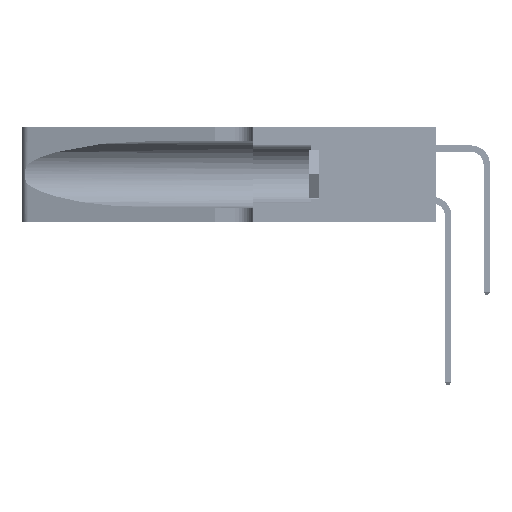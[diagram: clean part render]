
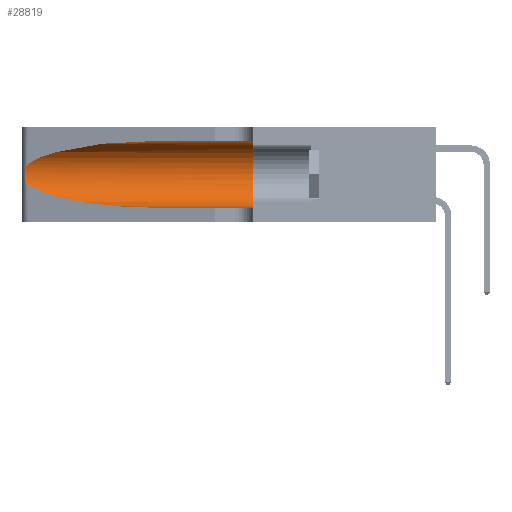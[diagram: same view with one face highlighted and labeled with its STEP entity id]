
A CAD part, left-side view. The second image highlights one B-rep face of the part: STEP entity #28819.
In plain terms, the highlighted cylindrical face has radius 3.308 mm (diameter 6.617 mm), a partial arc.
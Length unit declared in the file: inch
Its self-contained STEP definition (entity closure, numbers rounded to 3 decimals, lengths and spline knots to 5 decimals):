
#1353 = CARTESIAN_POINT ( 'NONE',  ( 0.1305, 0.72297, 0.05475 ) ) ;
#1608 = CARTESIAN_POINT ( 'NONE',  ( 0.25639, 1.23186, 0.15144 ) ) ;
#2017 = CARTESIAN_POINT ( 'NONE',  ( 0.1305, 0.35, 0.31525 ) ) ;
#2249 = ORIENTED_EDGE ( 'NONE', *, *, #4533, .F. ) ;
#2928 = DIRECTION ( 'NONE',  ( 0., 0., -1. ) ) ;
#4365 = CARTESIAN_POINT ( 'NONE',  ( 0.2373, 1.15595, 0.08982 ) ) ;
#4533 = EDGE_CURVE ( 'NONE', #17138, #28572, #42038, .T. ) ;
#5854 = CARTESIAN_POINT ( 'NONE',  ( 0.25487, 1.22718, 0.14631 ) ) ;
#6429 = EDGE_CURVE ( 'NONE', #27896, #28572, #28054, .T. ) ;
#7450 = ORIENTED_EDGE ( 'NONE', *, *, #48011, .T. ) ;
#9872 = CARTESIAN_POINT ( 'NONE',  ( 0.25639, 1.23184, 0.21858 ) ) ;
#12907 = CARTESIAN_POINT ( 'NONE',  ( 0.1305, 1.61858, 0.31525 ) ) ;
#14051 = CARTESIAN_POINT ( 'NONE',  ( 0.25854, 1.2359, 0.20912 ) ) ;
#16298 = AXIS2_PLACEMENT_3D ( 'NONE', #24358, #53357, #28524 ) ;
#16962 = CARTESIAN_POINT ( 'NONE',  ( 0.1305, 0.72297, 0.05475 ) ) ;
#17138 = VERTEX_POINT ( 'NONE', #2017 ) ;
#18266 = CARTESIAN_POINT ( 'NONE',  ( 0.26075, 1.23896, 0.19203 ) ) ;
#20744 = CARTESIAN_POINT ( 'NONE',  ( 0.25487, 1.22718, 0.22369 ) ) ;
#20755 = CYLINDRICAL_SURFACE ( 'NONE', #26564, 0.13025 ) ;
#20875 = ORIENTED_EDGE ( 'NONE', *, *, #33812, .T. ) ;
#22387 = CARTESIAN_POINT ( 'NONE',  ( 0.26017, 1.23833, 0.17102 ) ) ;
#23484 = EDGE_LOOP ( 'NONE', ( #20875, #49934, #7450, #38421, #2249, #41766 ) ) ;
#24358 = CARTESIAN_POINT ( 'NONE',  ( 0.1305, 0.35, 0.185 ) ) ;
#26370 = CARTESIAN_POINT ( 'NONE',  ( 0.25555, 1.22994, 0.2215 ) ) ;
#26554 = CARTESIAN_POINT ( 'NONE',  ( 0.25789, 1.23486, 0.15765 ) ) ;
#26564 = AXIS2_PLACEMENT_3D ( 'NONE', #48472, #31990, #2928 ) ;
#27896 = VERTEX_POINT ( 'NONE', #1353 ) ;
#28054 = LINE ( 'NONE', #49598, #48800 ) ;
#28524 = DIRECTION ( 'NONE',  ( 0., 0., 1. ) ) ;
#28572 = VERTEX_POINT ( 'NONE', #46867 ) ;
#28819 = ADVANCED_FACE ( 'NONE', ( #42798 ), #20755, .F. ) ;
#28870 = CARTESIAN_POINT ( 'NONE',  ( 0.1305, 0.72297, 0.31525 ) ) ;
#28943 = VERTEX_POINT ( 'NONE', #32700 ) ;
#29731 = EDGE_CURVE ( 'NONE', #28943, #17138, #52408, .T. ) ;
#30706 = CARTESIAN_POINT ( 'NONE',  ( 0.25555, 1.22993, 0.14849 ) ) ;
#31990 = DIRECTION ( 'NONE',  ( 0., -1., 0. ) ) ;
#32700 = CARTESIAN_POINT ( 'NONE',  ( 0.1305, 0.72297, 0.31525 ) ) ;
#33095 = DIRECTION ( 'NONE',  ( 0., -1., 0. ) ) ;
#33812 = EDGE_CURVE ( 'NONE', #28943, #36683, #44783, .T. ) ;
#36683 = VERTEX_POINT ( 'NONE', #49891 ) ;
#37570 = CARTESIAN_POINT ( 'NONE',  ( 0.25487, 1.22718, 0.14631 ) ) ;
#38421 = ORIENTED_EDGE ( 'NONE', *, *, #6429, .T. ) ;
#38883 = CARTESIAN_POINT ( 'NONE',  ( 0.25787, 1.23484, 0.2124 ) ) ;
#39419 = VERTEX_POINT ( 'NONE', #40006 ) ;
#40006 = CARTESIAN_POINT ( 'NONE',  ( 0.25487, 1.22718, 0.14631 ) ) ;
#40807 = B_SPLINE_CURVE_WITH_KNOTS ( 'NONE', 3,
 ( #51202, #26370, #9872, #38883, #14051, #43045, #18266, #47182, #22387, #51382, #26554, #1608, #30706, #5854 ),
 .UNSPECIFIED., .F., .F.,
 ( 4, 2, 2, 2, 2, 2, 4 ),
 ( 0., 0.00027, 0.00053, 0.00107, 0.0016, 0.00187, 0.00214 ),
 .UNSPECIFIED. ) ;
#41384 = VECTOR ( 'NONE', #41902, 39.37008 ) ;
#41759 = CARTESIAN_POINT ( 'NONE',  ( 0.18966, 0.96281, 0.05475 ) ) ;
#41766 = ORIENTED_EDGE ( 'NONE', *, *, #29731, .F. ) ;
#41902 = DIRECTION ( 'NONE',  ( 0., -1., 0. ) ) ;
#42038 = CIRCLE ( 'NONE', #16298, 0.13025 ) ;
#42798 = FACE_OUTER_BOUND ( 'NONE', #23484, .T. ) ;
#43045 = CARTESIAN_POINT ( 'NONE',  ( 0.26018, 1.23835, 0.19895 ) ) ;
#44783 =( BOUNDED_CURVE ( )  B_SPLINE_CURVE ( 3, ( #28870, #53714, #45528, #20744 ),
 .UNSPECIFIED., .F., .T. ) 
 B_SPLINE_CURVE_WITH_KNOTS ( ( 4, 4 ),
 ( 1.5708, 2.84003 ),
 .UNSPECIFIED. ) 
 CURVE ( )  GEOMETRIC_REPRESENTATION_ITEM ( )  RATIONAL_B_SPLINE_CURVE ( ( 1., 0.87, 0.87, 1. ) ) 
 REPRESENTATION_ITEM ( '' )  );
#45528 = CARTESIAN_POINT ( 'NONE',  ( 0.2373, 1.15595, 0.28018 ) ) ;
#46867 = CARTESIAN_POINT ( 'NONE',  ( 0.1305, 0.35, 0.05475 ) ) ;
#47182 = CARTESIAN_POINT ( 'NONE',  ( 0.26075, 1.23896, 0.178 ) ) ;
#48011 = EDGE_CURVE ( 'NONE', #39419, #27896, #50439, .T. ) ;
#48472 = CARTESIAN_POINT ( 'NONE',  ( 0.1305, 1.61858, 0.185 ) ) ;
#48800 = VECTOR ( 'NONE', #33095, 39.37008 ) ;
#49598 = CARTESIAN_POINT ( 'NONE',  ( 0.1305, 1.61858, 0.05475 ) ) ;
#49891 = CARTESIAN_POINT ( 'NONE',  ( 0.25487, 1.22718, 0.22369 ) ) ;
#49897 = EDGE_CURVE ( 'NONE', #36683, #39419, #40807, .T. ) ;
#49934 = ORIENTED_EDGE ( 'NONE', *, *, #49897, .T. ) ;
#50439 =( BOUNDED_CURVE ( )  B_SPLINE_CURVE ( 3, ( #37570, #4365, #41759, #16962 ),
 .UNSPECIFIED., .F., .F. ) 
 B_SPLINE_CURVE_WITH_KNOTS ( ( 4, 4 ),
 ( 3.44316, 4.71239 ),
 .UNSPECIFIED. ) 
 CURVE ( )  GEOMETRIC_REPRESENTATION_ITEM ( )  RATIONAL_B_SPLINE_CURVE ( ( 1., 0.87, 0.87, 1. ) ) 
 REPRESENTATION_ITEM ( '' )  );
#51202 = CARTESIAN_POINT ( 'NONE',  ( 0.25487, 1.22718, 0.22369 ) ) ;
#51382 = CARTESIAN_POINT ( 'NONE',  ( 0.25856, 1.23593, 0.16098 ) ) ;
#52408 = LINE ( 'NONE', #12907, #41384 ) ;
#53357 = DIRECTION ( 'NONE',  ( 0., 1., 0. ) ) ;
#53714 = CARTESIAN_POINT ( 'NONE',  ( 0.18966, 0.96281, 0.31525 ) ) ;
